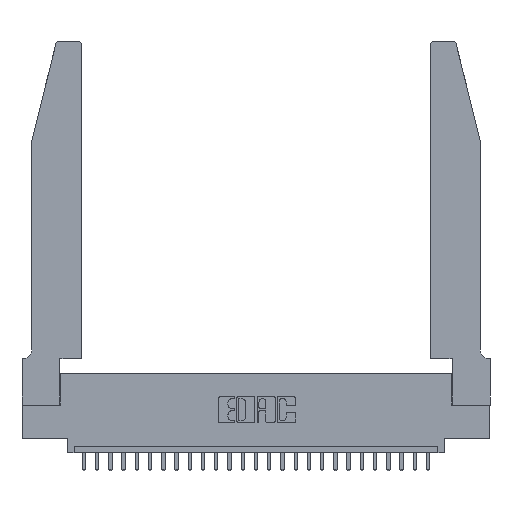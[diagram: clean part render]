
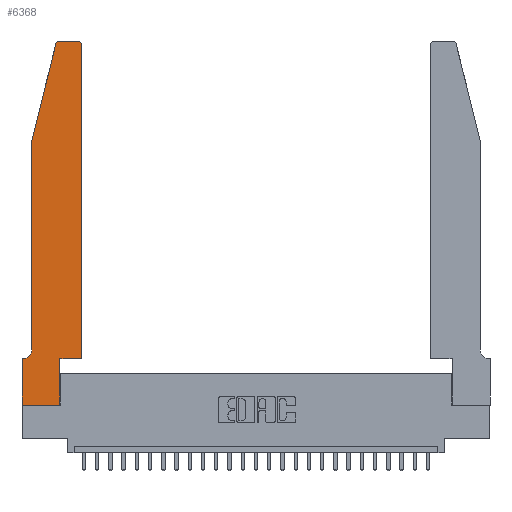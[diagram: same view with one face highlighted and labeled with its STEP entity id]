
A CAD part, top view. The second image highlights one B-rep face of the part: STEP entity #6368.
In plain terms, the highlighted planar face has unit normal (0, 0, 1).
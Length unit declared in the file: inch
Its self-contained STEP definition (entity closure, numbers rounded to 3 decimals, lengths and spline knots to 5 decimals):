
#122 = VERTEX_POINT ( 'NONE', #23564 ) ;
#301 = VECTOR ( 'NONE', #1086, 39.37008 ) ;
#457 = AXIS2_PLACEMENT_3D ( 'NONE', #17507, #15383, #9009 ) ;
#727 = DIRECTION ( 'NONE',  ( 1., 0., 0. ) ) ;
#1086 = DIRECTION ( 'NONE',  ( 0., 1., 0. ) ) ;
#1301 = EDGE_CURVE ( 'NONE', #23450, #2876, #23985, .T. ) ;
#1470 = LINE ( 'NONE', #20784, #14048 ) ;
#1883 = CARTESIAN_POINT ( 'NONE',  ( 0.0755, 0.35, 0.37 ) ) ;
#2432 = CARTESIAN_POINT ( 'NONE',  ( 0.0755, 2., 0.37 ) ) ;
#2725 = CARTESIAN_POINT ( 'NONE',  ( 0., 0.35, 0.37 ) ) ;
#2768 = VECTOR ( 'NONE', #3719, 39.37008 ) ;
#2876 = VERTEX_POINT ( 'NONE', #8847 ) ;
#3279 = EDGE_CURVE ( 'NONE', #26686, #23844, #1470, .T. ) ;
#3385 = VERTEX_POINT ( 'NONE', #25335 ) ;
#3428 = DIRECTION ( 'NONE',  ( 1., 0., 0. ) ) ;
#3577 = VECTOR ( 'NONE', #7679, 39.37008 ) ;
#3719 = DIRECTION ( 'NONE',  ( -1., 0., 0. ) ) ;
#3774 = EDGE_CURVE ( 'NONE', #2876, #8481, #4451, .T. ) ;
#3796 = ORIENTED_EDGE ( 'NONE', *, *, #8531, .T. ) ;
#4025 = DIRECTION ( 'NONE',  ( -1., 0., 0. ) ) ;
#4343 = DIRECTION ( 'NONE',  ( 1., 0., 0. ) ) ;
#4451 = LINE ( 'NONE', #9900, #2768 ) ;
#4616 = VERTEX_POINT ( 'NONE', #25642 ) ;
#5384 = VERTEX_POINT ( 'NONE', #17884 ) ;
#5550 = CARTESIAN_POINT ( 'NONE',  ( 0., 0., 0.37 ) ) ;
#5737 = DIRECTION ( 'NONE',  ( 0., 0., 1. ) ) ;
#6112 = ORIENTED_EDGE ( 'NONE', *, *, #1301, .T. ) ;
#6368 = ADVANCED_FACE ( 'NONE', ( #10951 ), #13252, .T. ) ;
#6750 = ORIENTED_EDGE ( 'NONE', *, *, #11889, .T. ) ;
#6777 = EDGE_CURVE ( 'NONE', #8481, #26686, #18877, .T. ) ;
#7679 = DIRECTION ( 'NONE',  ( 0., -1., 0. ) ) ;
#7850 = CARTESIAN_POINT ( 'NONE',  ( 0.4505, 0.35, 0.37 ) ) ;
#8010 = EDGE_CURVE ( 'NONE', #13071, #4616, #20421, .T. ) ;
#8175 = DIRECTION ( 'NONE',  ( -0.239, -0.971, 0. ) ) ;
#8481 = VERTEX_POINT ( 'NONE', #20964 ) ;
#8531 = EDGE_CURVE ( 'NONE', #122, #13071, #10220, .T. ) ;
#8847 = CARTESIAN_POINT ( 'NONE',  ( 0.4205, 2.75, 0.37 ) ) ;
#8887 = DIRECTION ( 'NONE',  ( 1., 0., 0. ) ) ;
#8911 = DIRECTION ( 'NONE',  ( 0., 0., -1. ) ) ;
#9009 = DIRECTION ( 'NONE',  ( 1., 0., 0. ) ) ;
#9029 = AXIS2_PLACEMENT_3D ( 'NONE', #25517, #8911, #23599 ) ;
#9325 = CARTESIAN_POINT ( 'NONE',  ( 0., 0., 0.37 ) ) ;
#9900 = CARTESIAN_POINT ( 'NONE',  ( 0.2605, 2.75, 0.37 ) ) ;
#10220 = LINE ( 'NONE', #1883, #14209 ) ;
#10595 = VERTEX_POINT ( 'NONE', #24715 ) ;
#10607 = CARTESIAN_POINT ( 'NONE',  ( 0.2865, 0., 0.37 ) ) ;
#10808 = EDGE_CURVE ( 'NONE', #11605, #10595, #13059, .T. ) ;
#10951 = FACE_OUTER_BOUND ( 'NONE', #16298, .T. ) ;
#11605 = VERTEX_POINT ( 'NONE', #10607 ) ;
#11852 = EDGE_CURVE ( 'NONE', #5384, #122, #20251, .T. ) ;
#11889 = EDGE_CURVE ( 'NONE', #23844, #5384, #17984, .T. ) ;
#11921 = CARTESIAN_POINT ( 'NONE',  ( 0.4205, 2.72, 0.37 ) ) ;
#12427 = AXIS2_PLACEMENT_3D ( 'NONE', #11921, #5737, #3428 ) ;
#12428 = ORIENTED_EDGE ( 'NONE', *, *, #10808, .T. ) ;
#12872 = CARTESIAN_POINT ( 'NONE',  ( 0.284, 2.72, 0.37 ) ) ;
#12873 = EDGE_CURVE ( 'NONE', #3385, #23450, #23986, .T. ) ;
#12991 = CARTESIAN_POINT ( 'NONE',  ( 0.2865, 0.35, 0.37 ) ) ;
#13059 = LINE ( 'NONE', #12991, #23551 ) ;
#13071 = VERTEX_POINT ( 'NONE', #2725 ) ;
#13252 = PLANE ( 'NONE',  #457 ) ;
#13270 = ORIENTED_EDGE ( 'NONE', *, *, #8010, .T. ) ;
#14048 = VECTOR ( 'NONE', #8175, 39.37008 ) ;
#14209 = VECTOR ( 'NONE', #4025, 39.37008 ) ;
#14917 = ORIENTED_EDGE ( 'NONE', *, *, #3279, .T. ) ;
#15015 = ORIENTED_EDGE ( 'NONE', *, *, #11852, .T. ) ;
#15383 = DIRECTION ( 'NONE',  ( 0., 0., 1. ) ) ;
#15850 = CARTESIAN_POINT ( 'NONE',  ( 0.0755, 2., 0.37 ) ) ;
#16298 = EDGE_LOOP ( 'NONE', ( #20012, #25338, #14917, #6750, #15015, #3796, #13270, #23412, #12428, #23488, #20182, #6112 ) ) ;
#16793 = CARTESIAN_POINT ( 'NONE',  ( 0.4505, 2.72, 0.37 ) ) ;
#17125 = VECTOR ( 'NONE', #4343, 39.37008 ) ;
#17507 = CARTESIAN_POINT ( 'NONE',  ( 0., 0.35, 0.37 ) ) ;
#17884 = CARTESIAN_POINT ( 'NONE',  ( 0.0755, 0.42, 0.37 ) ) ;
#17984 = LINE ( 'NONE', #2432, #19285 ) ;
#18470 = LINE ( 'NONE', #25292, #17125 ) ;
#18701 = AXIS2_PLACEMENT_3D ( 'NONE', #12872, #21470, #8887 ) ;
#18877 = CIRCLE ( 'NONE', #18701, 0.03 ) ;
#19285 = VECTOR ( 'NONE', #19613, 39.37008 ) ;
#19613 = DIRECTION ( 'NONE',  ( 0., -1., 0. ) ) ;
#19717 = EDGE_CURVE ( 'NONE', #10595, #3385, #18470, .T. ) ;
#20012 = ORIENTED_EDGE ( 'NONE', *, *, #3774, .T. ) ;
#20059 = LINE ( 'NONE', #9325, #21032 ) ;
#20182 = ORIENTED_EDGE ( 'NONE', *, *, #12873, .T. ) ;
#20251 = CIRCLE ( 'NONE', #9029, 0.07 ) ;
#20421 = LINE ( 'NONE', #5550, #3577 ) ;
#20784 = CARTESIAN_POINT ( 'NONE',  ( 0.0755, 2., 0.37 ) ) ;
#20788 = CARTESIAN_POINT ( 'NONE',  ( 0.25487, 2.72718, 0.37 ) ) ;
#20964 = CARTESIAN_POINT ( 'NONE',  ( 0.284, 2.75, 0.37 ) ) ;
#21032 = VECTOR ( 'NONE', #727, 39.37008 ) ;
#21470 = DIRECTION ( 'NONE',  ( 0., 0., 1. ) ) ;
#23412 = ORIENTED_EDGE ( 'NONE', *, *, #25976, .T. ) ;
#23450 = VERTEX_POINT ( 'NONE', #16793 ) ;
#23488 = ORIENTED_EDGE ( 'NONE', *, *, #19717, .T. ) ;
#23551 = VECTOR ( 'NONE', #25620, 39.37008 ) ;
#23564 = CARTESIAN_POINT ( 'NONE',  ( 0.0055, 0.35, 0.37 ) ) ;
#23599 = DIRECTION ( 'NONE',  ( -1., 0., 0. ) ) ;
#23844 = VERTEX_POINT ( 'NONE', #15850 ) ;
#23985 = CIRCLE ( 'NONE', #12427, 0.03 ) ;
#23986 = LINE ( 'NONE', #7850, #301 ) ;
#24715 = CARTESIAN_POINT ( 'NONE',  ( 0.2865, 0.35, 0.37 ) ) ;
#25292 = CARTESIAN_POINT ( 'NONE',  ( 0.4505, 0.35, 0.37 ) ) ;
#25335 = CARTESIAN_POINT ( 'NONE',  ( 0.4505, 0.35, 0.37 ) ) ;
#25338 = ORIENTED_EDGE ( 'NONE', *, *, #6777, .T. ) ;
#25517 = CARTESIAN_POINT ( 'NONE',  ( 0.0055, 0.42, 0.37 ) ) ;
#25620 = DIRECTION ( 'NONE',  ( 0., 1., 0. ) ) ;
#25642 = CARTESIAN_POINT ( 'NONE',  ( 0., 0., 0.37 ) ) ;
#25976 = EDGE_CURVE ( 'NONE', #4616, #11605, #20059, .T. ) ;
#26686 = VERTEX_POINT ( 'NONE', #20788 ) ;
